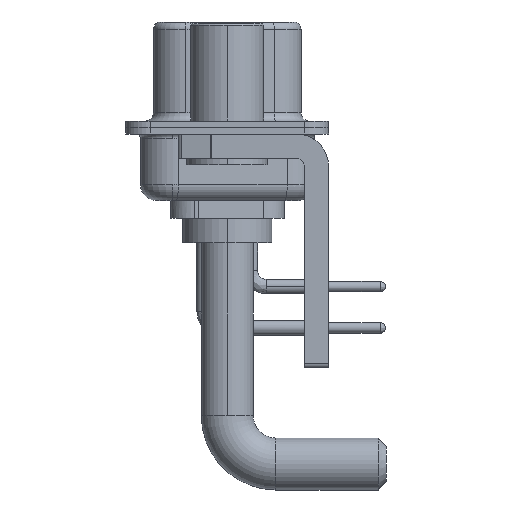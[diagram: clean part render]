
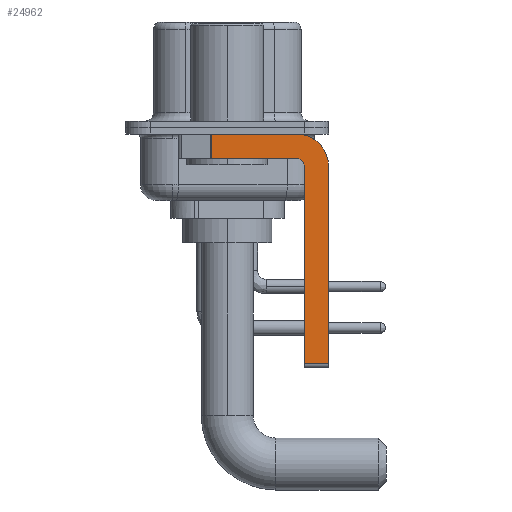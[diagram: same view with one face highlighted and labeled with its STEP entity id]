
A CAD part, left-side view. The second image highlights one B-rep face of the part: STEP entity #24962.
In plain terms, the highlighted planar face has unit normal (-1, 0, 0).
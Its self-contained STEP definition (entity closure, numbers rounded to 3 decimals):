
#110 = VERTEX_POINT ( 'NONE', #23701 ) ;
#337 = CARTESIAN_POINT ( 'NONE',  ( -2.9, -4.25, -2.4 ) ) ;
#364 = CIRCLE ( 'NONE', #17499, 0.5 ) ;
#415 = VERTEX_POINT ( 'NONE', #23400 ) ;
#2099 = VECTOR ( 'NONE', #26977, 1000. ) ;
#2418 = AXIS2_PLACEMENT_3D ( 'NONE', #337, #12882, #15193 ) ;
#2447 = CARTESIAN_POINT ( 'NONE',  ( -2.9, 0.978, -1.9 ) ) ;
#2582 = CARTESIAN_POINT ( 'NONE',  ( -2.9, -4.25, -2.4 ) ) ;
#2792 = EDGE_CURVE ( 'NONE', #25037, #110, #15476, .T. ) ;
#3769 = VECTOR ( 'NONE', #21949, 1000. ) ;
#4119 = DIRECTION ( 'NONE',  ( 0., 0., -1. ) ) ;
#4416 = DIRECTION ( 'NONE',  ( 0., 0., 1. ) ) ;
#5086 = ORIENTED_EDGE ( 'NONE', *, *, #12618, .F. ) ;
#6010 = EDGE_CURVE ( 'NONE', #8590, #110, #27111, .T. ) ;
#6651 = CARTESIAN_POINT ( 'NONE',  ( -2.9, 0.978, -0.4 ) ) ;
#6715 = CARTESIAN_POINT ( 'NONE',  ( -2.9, 0.978, -1.9 ) ) ;
#7263 = CARTESIAN_POINT ( 'NONE',  ( -2.9, -4.75, -2.4 ) ) ;
#7273 = CARTESIAN_POINT ( 'NONE',  ( -2.9, -4.25, -0.4 ) ) ;
#7884 = LINE ( 'NONE', #24547, #22328 ) ;
#8550 = LINE ( 'NONE', #23414, #17632 ) ;
#8582 = CIRCLE ( 'NONE', #2418, 2. ) ;
#8590 = VERTEX_POINT ( 'NONE', #22697 ) ;
#8966 = ORIENTED_EDGE ( 'NONE', *, *, #18806, .T. ) ;
#9372 = ORIENTED_EDGE ( 'NONE', *, *, #6010, .T. ) ;
#9700 = EDGE_LOOP ( 'NONE', ( #5086, #8966, #20573, #11962, #12780, #9372, #22825, #18688 ) ) ;
#9949 = DIRECTION ( 'NONE',  ( 0., -1., 0. ) ) ;
#10260 = PLANE ( 'NONE',  #18460 ) ;
#10483 = EDGE_CURVE ( 'NONE', #22374, #25037, #8582, .T. ) ;
#10891 = DIRECTION ( 'NONE',  ( 0., 1., 0. ) ) ;
#11962 = ORIENTED_EDGE ( 'NONE', *, *, #22216, .F. ) ;
#12465 = CARTESIAN_POINT ( 'NONE',  ( -2.9, -6.25, -2.4 ) ) ;
#12511 = CARTESIAN_POINT ( 'NONE',  ( -2.9, -4.25, -14.55 ) ) ;
#12618 = EDGE_CURVE ( 'NONE', #17257, #22374, #7884, .T. ) ;
#12780 = ORIENTED_EDGE ( 'NONE', *, *, #16337, .F. ) ;
#12818 = LINE ( 'NONE', #19000, #21743 ) ;
#12882 = DIRECTION ( 'NONE',  ( 1., 0., 0. ) ) ;
#15193 = DIRECTION ( 'NONE',  ( 0., 0., -1. ) ) ;
#15476 = LINE ( 'NONE', #17254, #3769 ) ;
#15985 = VECTOR ( 'NONE', #4119, 1000. ) ;
#16300 = CARTESIAN_POINT ( 'NONE',  ( -2.9, -4.25, -2.4 ) ) ;
#16337 = EDGE_CURVE ( 'NONE', #8590, #24385, #8550, .T. ) ;
#17164 = DIRECTION ( 'NONE',  ( -1., 0., 0. ) ) ;
#17254 = CARTESIAN_POINT ( 'NONE',  ( -2.9, -6.25, -2.4 ) ) ;
#17257 = VERTEX_POINT ( 'NONE', #6651 ) ;
#17499 = AXIS2_PLACEMENT_3D ( 'NONE', #2582, #17164, #25587 ) ;
#17632 = VECTOR ( 'NONE', #4416, 1000. ) ;
#18460 = AXIS2_PLACEMENT_3D ( 'NONE', #16300, #24714, #20853 ) ;
#18688 = ORIENTED_EDGE ( 'NONE', *, *, #10483, .F. ) ;
#18806 = EDGE_CURVE ( 'NONE', #17257, #23024, #27127, .T. ) ;
#19000 = CARTESIAN_POINT ( 'NONE',  ( -2.9, -4.25, -1.9 ) ) ;
#19776 = EDGE_CURVE ( 'NONE', #415, #23024, #12818, .T. ) ;
#20573 = ORIENTED_EDGE ( 'NONE', *, *, #19776, .F. ) ;
#20853 = DIRECTION ( 'NONE',  ( 0., 0., -1. ) ) ;
#21743 = VECTOR ( 'NONE', #10891, 1000. ) ;
#21949 = DIRECTION ( 'NONE',  ( 0., 0., -1. ) ) ;
#22216 = EDGE_CURVE ( 'NONE', #24385, #415, #364, .T. ) ;
#22328 = VECTOR ( 'NONE', #9949, 1000. ) ;
#22374 = VERTEX_POINT ( 'NONE', #7273 ) ;
#22697 = CARTESIAN_POINT ( 'NONE',  ( -2.9, -4.75, -14.55 ) ) ;
#22825 = ORIENTED_EDGE ( 'NONE', *, *, #2792, .F. ) ;
#23024 = VERTEX_POINT ( 'NONE', #2447 ) ;
#23400 = CARTESIAN_POINT ( 'NONE',  ( -2.9, -4.25, -1.9 ) ) ;
#23414 = CARTESIAN_POINT ( 'NONE',  ( -2.9, -4.75, -14.8 ) ) ;
#23701 = CARTESIAN_POINT ( 'NONE',  ( -2.9, -6.25, -14.55 ) ) ;
#24385 = VERTEX_POINT ( 'NONE', #7263 ) ;
#24547 = CARTESIAN_POINT ( 'NONE',  ( -2.9, 3., -0.4 ) ) ;
#24714 = DIRECTION ( 'NONE',  ( 1., 0., 0. ) ) ;
#24962 = ADVANCED_FACE ( 'NONE', ( #27208 ), #10260, .F. ) ;
#25037 = VERTEX_POINT ( 'NONE', #12465 ) ;
#25587 = DIRECTION ( 'NONE',  ( 0., 0., 1. ) ) ;
#26977 = DIRECTION ( 'NONE',  ( 0., -1., 0. ) ) ;
#27111 = LINE ( 'NONE', #12511, #2099 ) ;
#27127 = LINE ( 'NONE', #6715, #15985 ) ;
#27208 = FACE_OUTER_BOUND ( 'NONE', #9700, .T. ) ;
